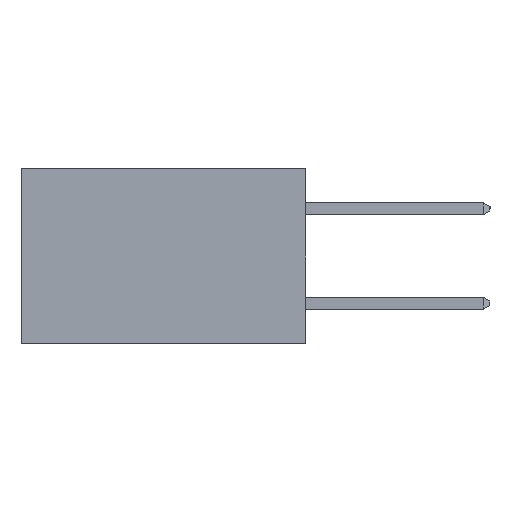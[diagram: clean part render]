
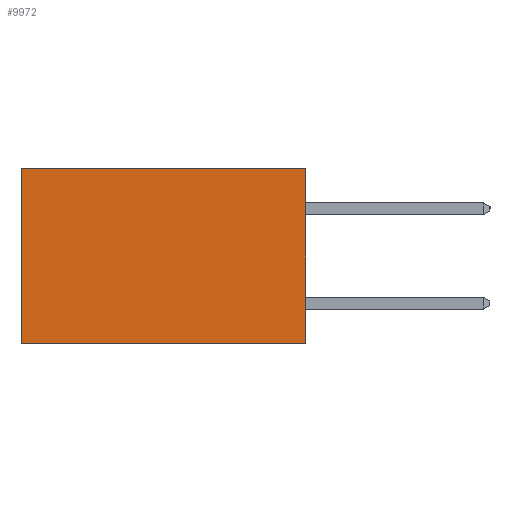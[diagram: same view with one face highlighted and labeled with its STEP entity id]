
A CAD part, left-side view. The second image highlights one B-rep face of the part: STEP entity #9972.
In plain terms, the highlighted planar face has unit normal (-1, 0, 0).
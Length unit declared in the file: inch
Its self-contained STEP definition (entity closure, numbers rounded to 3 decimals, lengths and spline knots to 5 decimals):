
#278 = CARTESIAN_POINT ( 'NONE',  ( 0.2615, 0., -0.37 ) ) ;
#889 = VECTOR ( 'NONE', #10388, 39.37008 ) ;
#1351 = LINE ( 'NONE', #278, #12427 ) ;
#1387 = VERTEX_POINT ( 'NONE', #11435 ) ;
#1488 = DIRECTION ( 'NONE',  ( 1., 0., 0. ) ) ;
#1627 = ORIENTED_EDGE ( 'NONE', *, *, #9774, .F. ) ;
#1724 = VECTOR ( 'NONE', #7597, 39.37008 ) ;
#2021 = CARTESIAN_POINT ( 'NONE',  ( 0.2615, 0.6, -0.37 ) ) ;
#2095 = DIRECTION ( 'NONE',  ( 0., 0., -1. ) ) ;
#2565 = CARTESIAN_POINT ( 'NONE',  ( 0.2615, 0., 0. ) ) ;
#2863 = AXIS2_PLACEMENT_3D ( 'NONE', #11835, #1488, #11971 ) ;
#3218 = CARTESIAN_POINT ( 'NONE',  ( 0.2615, 0.6, -0.37 ) ) ;
#3388 = CARTESIAN_POINT ( 'NONE',  ( 0.2615, 0.6, 0. ) ) ;
#3663 = FACE_OUTER_BOUND ( 'NONE', #4615, .T. ) ;
#4615 = EDGE_LOOP ( 'NONE', ( #10057, #11594, #1627, #9162 ) ) ;
#4718 = EDGE_CURVE ( 'NONE', #1387, #6042, #12413, .T. ) ;
#5289 = LINE ( 'NONE', #2021, #889 ) ;
#5627 = LINE ( 'NONE', #2565, #1724 ) ;
#6042 = VERTEX_POINT ( 'NONE', #3218 ) ;
#6702 = CARTESIAN_POINT ( 'NONE',  ( 0.2615, 0., 0. ) ) ;
#7597 = DIRECTION ( 'NONE',  ( 0., 1., 0. ) ) ;
#7817 = PLANE ( 'NONE',  #2863 ) ;
#8270 = CARTESIAN_POINT ( 'NONE',  ( 0.2615, 0., -0.37 ) ) ;
#8301 = EDGE_CURVE ( 'NONE', #9696, #6042, #5289, .T. ) ;
#9162 = ORIENTED_EDGE ( 'NONE', *, *, #11632, .T. ) ;
#9482 = DIRECTION ( 'NONE',  ( 0., 1., 0. ) ) ;
#9696 = VERTEX_POINT ( 'NONE', #3388 ) ;
#9774 = EDGE_CURVE ( 'NONE', #12552, #1387, #1351, .T. ) ;
#9972 = ADVANCED_FACE ( 'NONE', ( #3663 ), #7817, .F. ) ;
#10057 = ORIENTED_EDGE ( 'NONE', *, *, #8301, .T. ) ;
#10388 = DIRECTION ( 'NONE',  ( 0., 0., -1. ) ) ;
#11391 = VECTOR ( 'NONE', #9482, 39.37008 ) ;
#11435 = CARTESIAN_POINT ( 'NONE',  ( 0.2615, 0., -0.37 ) ) ;
#11594 = ORIENTED_EDGE ( 'NONE', *, *, #4718, .F. ) ;
#11632 = EDGE_CURVE ( 'NONE', #12552, #9696, #5627, .T. ) ;
#11835 = CARTESIAN_POINT ( 'NONE',  ( 0.2615, 0., -0.37 ) ) ;
#11971 = DIRECTION ( 'NONE',  ( 0., 0., -1. ) ) ;
#12413 = LINE ( 'NONE', #8270, #11391 ) ;
#12427 = VECTOR ( 'NONE', #2095, 39.37008 ) ;
#12552 = VERTEX_POINT ( 'NONE', #6702 ) ;
